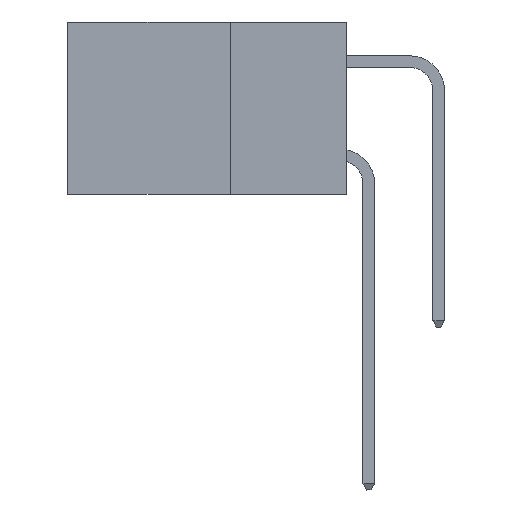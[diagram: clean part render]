
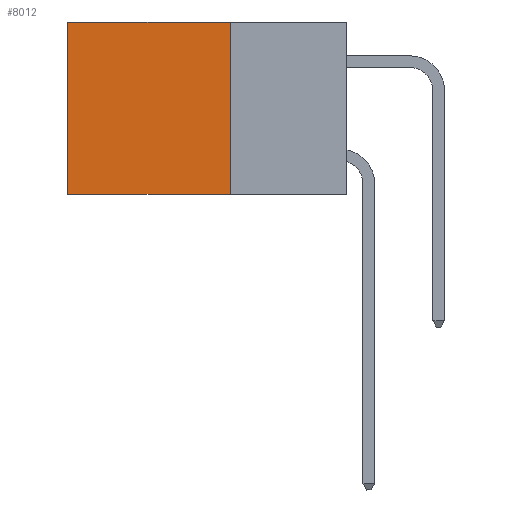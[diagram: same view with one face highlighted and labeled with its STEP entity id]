
A CAD part, left-side view. The second image highlights one B-rep face of the part: STEP entity #8012.
In plain terms, the highlighted planar face has unit normal (-1, 0, 0).
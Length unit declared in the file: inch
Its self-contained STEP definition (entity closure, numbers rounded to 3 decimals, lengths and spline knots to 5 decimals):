
#733 = VERTEX_POINT ( 'NONE', #2081 ) ;
#882 = AXIS2_PLACEMENT_3D ( 'NONE', #10055, #11812, #6693 ) ;
#1196 = EDGE_LOOP ( 'NONE', ( #21143, #22039, #7152, #12069 ) ) ;
#1279 = DIRECTION ( 'NONE',  ( 0., 1., 0. ) ) ;
#2081 = CARTESIAN_POINT ( 'NONE',  ( 0.2875, 0.6, -0.37 ) ) ;
#3186 = FACE_OUTER_BOUND ( 'NONE', #1196, .T. ) ;
#3441 = LINE ( 'NONE', #22629, #19481 ) ;
#3700 = VERTEX_POINT ( 'NONE', #14537 ) ;
#4883 = VECTOR ( 'NONE', #16141, 39.37008 ) ;
#6693 = DIRECTION ( 'NONE',  ( 0., 0., -1. ) ) ;
#7152 = ORIENTED_EDGE ( 'NONE', *, *, #16202, .F. ) ;
#8012 = ADVANCED_FACE ( 'NONE', ( #3186 ), #18834, .F. ) ;
#9543 = EDGE_CURVE ( 'NONE', #3700, #10987, #3441, .T. ) ;
#9694 = CARTESIAN_POINT ( 'NONE',  ( 0.2875, 0.25, -0.37 ) ) ;
#10055 = CARTESIAN_POINT ( 'NONE',  ( 0.2875, 0.25, 0. ) ) ;
#10987 = VERTEX_POINT ( 'NONE', #15509 ) ;
#11812 = DIRECTION ( 'NONE',  ( 1., 0., 0. ) ) ;
#12069 = ORIENTED_EDGE ( 'NONE', *, *, #9543, .T. ) ;
#12281 = VERTEX_POINT ( 'NONE', #19954 ) ;
#13596 = LINE ( 'NONE', #20414, #16303 ) ;
#13691 = VECTOR ( 'NONE', #1279, 39.37008 ) ;
#14180 = EDGE_CURVE ( 'NONE', #10987, #733, #20684, .T. ) ;
#14378 = CARTESIAN_POINT ( 'NONE',  ( 0.2875, 0.6, 0. ) ) ;
#14537 = CARTESIAN_POINT ( 'NONE',  ( 0.2875, 0.25, 0. ) ) ;
#14927 = DIRECTION ( 'NONE',  ( 0., 0., -1. ) ) ;
#15509 = CARTESIAN_POINT ( 'NONE',  ( 0.2875, 0.6, 0. ) ) ;
#15620 = DIRECTION ( 'NONE',  ( 0., 1., 0. ) ) ;
#16141 = DIRECTION ( 'NONE',  ( 0., 0., -1. ) ) ;
#16202 = EDGE_CURVE ( 'NONE', #3700, #12281, #13596, .T. ) ;
#16303 = VECTOR ( 'NONE', #14927, 39.37008 ) ;
#18652 = LINE ( 'NONE', #9694, #13691 ) ;
#18834 = PLANE ( 'NONE',  #882 ) ;
#19481 = VECTOR ( 'NONE', #15620, 39.37008 ) ;
#19624 = EDGE_CURVE ( 'NONE', #12281, #733, #18652, .T. ) ;
#19954 = CARTESIAN_POINT ( 'NONE',  ( 0.2875, 0.25, -0.37 ) ) ;
#20414 = CARTESIAN_POINT ( 'NONE',  ( 0.2875, 0.25, 0. ) ) ;
#20684 = LINE ( 'NONE', #14378, #4883 ) ;
#21143 = ORIENTED_EDGE ( 'NONE', *, *, #14180, .T. ) ;
#22039 = ORIENTED_EDGE ( 'NONE', *, *, #19624, .F. ) ;
#22629 = CARTESIAN_POINT ( 'NONE',  ( 0.2875, 0.25, 0. ) ) ;
